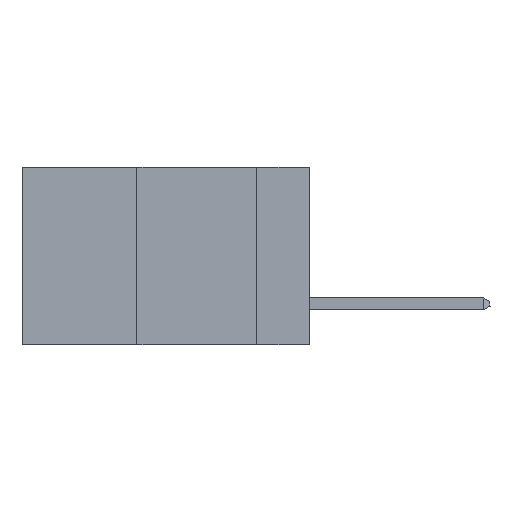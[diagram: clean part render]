
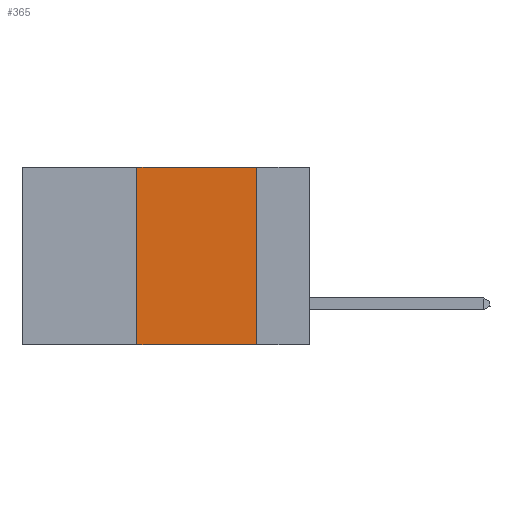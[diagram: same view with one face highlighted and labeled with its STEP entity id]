
A CAD part, left-side view. The second image highlights one B-rep face of the part: STEP entity #365.
In plain terms, the highlighted planar face has unit normal (-1, 0, 0).
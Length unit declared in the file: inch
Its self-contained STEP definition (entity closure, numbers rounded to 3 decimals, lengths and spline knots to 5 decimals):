
#188 = FACE_OUTER_BOUND ( 'NONE', #6446, .T. ) ;
#365 = ADVANCED_FACE ( 'NONE', ( #188 ), #8962, .F. ) ;
#868 = ORIENTED_EDGE ( 'NONE', *, *, #14551, .F. ) ;
#1066 = LINE ( 'NONE', #7464, #4108 ) ;
#1386 = VERTEX_POINT ( 'NONE', #18162 ) ;
#3491 = CARTESIAN_POINT ( 'NONE',  ( 0., 0.11, 0. ) ) ;
#3554 = DIRECTION ( 'NONE',  ( 0., 0., -1. ) ) ;
#4054 = VECTOR ( 'NONE', #8989, 39.37008 ) ;
#4108 = VECTOR ( 'NONE', #13613, 39.37008 ) ;
#4371 = CARTESIAN_POINT ( 'NONE',  ( 0., 0.36, -0.37 ) ) ;
#4460 = CARTESIAN_POINT ( 'NONE',  ( 0., 0.6, 0. ) ) ;
#4486 = CARTESIAN_POINT ( 'NONE',  ( 0., 0.6, -0.37 ) ) ;
#4899 = VECTOR ( 'NONE', #17823, 39.37008 ) ;
#5255 = VERTEX_POINT ( 'NONE', #4371 ) ;
#6209 = CARTESIAN_POINT ( 'NONE',  ( 0., 0.11, -0.37 ) ) ;
#6446 = EDGE_LOOP ( 'NONE', ( #13585, #10743, #868, #16770 ) ) ;
#7076 = LINE ( 'NONE', #4486, #4054 ) ;
#7464 = CARTESIAN_POINT ( 'NONE',  ( 0., 0.6, 0. ) ) ;
#7691 = LINE ( 'NONE', #11622, #4899 ) ;
#8575 = EDGE_CURVE ( 'NONE', #1386, #9568, #1066, .T. ) ;
#8962 = PLANE ( 'NONE',  #18822 ) ;
#8989 = DIRECTION ( 'NONE',  ( 0., -1., 0. ) ) ;
#9568 = VERTEX_POINT ( 'NONE', #15970 ) ;
#10743 = ORIENTED_EDGE ( 'NONE', *, *, #8575, .F. ) ;
#11622 = CARTESIAN_POINT ( 'NONE',  ( 0., 0.36, 0. ) ) ;
#13482 = DIRECTION ( 'NONE',  ( 1., 0., 0. ) ) ;
#13585 = ORIENTED_EDGE ( 'NONE', *, *, #17429, .F. ) ;
#13613 = DIRECTION ( 'NONE',  ( 0., -1., 0. ) ) ;
#14551 = EDGE_CURVE ( 'NONE', #5255, #1386, #7691, .T. ) ;
#14615 = LINE ( 'NONE', #3491, #15576 ) ;
#15576 = VECTOR ( 'NONE', #3554, 39.37008 ) ;
#15970 = CARTESIAN_POINT ( 'NONE',  ( 0., 0.11, 0. ) ) ;
#16770 = ORIENTED_EDGE ( 'NONE', *, *, #18034, .T. ) ;
#17429 = EDGE_CURVE ( 'NONE', #9568, #18170, #14615, .T. ) ;
#17823 = DIRECTION ( 'NONE',  ( 0., 0., 1. ) ) ;
#18034 = EDGE_CURVE ( 'NONE', #5255, #18170, #7076, .T. ) ;
#18162 = CARTESIAN_POINT ( 'NONE',  ( 0., 0.36, 0. ) ) ;
#18170 = VERTEX_POINT ( 'NONE', #6209 ) ;
#18200 = DIRECTION ( 'NONE',  ( 0., 0., -1. ) ) ;
#18822 = AXIS2_PLACEMENT_3D ( 'NONE', #4460, #13482, #18200 ) ;
